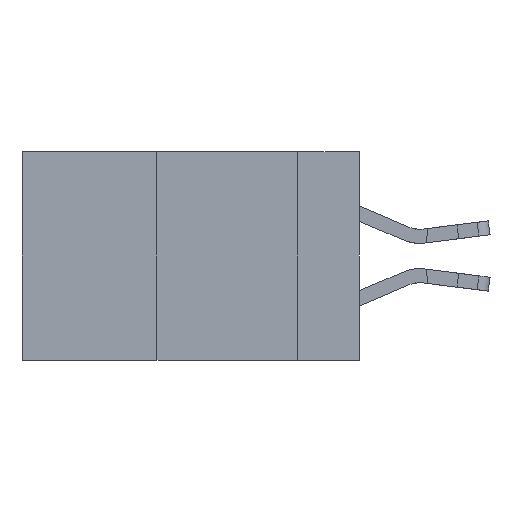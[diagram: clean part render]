
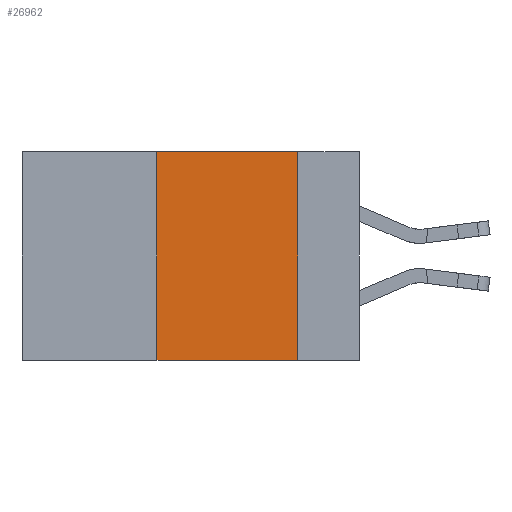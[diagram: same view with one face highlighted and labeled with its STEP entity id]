
A CAD part, left-side view. The second image highlights one B-rep face of the part: STEP entity #26962.
In plain terms, the highlighted planar face has unit normal (-1, 0, 0).
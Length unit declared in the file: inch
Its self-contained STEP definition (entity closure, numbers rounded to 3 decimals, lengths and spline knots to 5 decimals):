
#1200 = AXIS2_PLACEMENT_3D ( 'NONE', #20903, #7798, #16596 ) ;
#1503 = EDGE_CURVE ( 'NONE', #26457, #20012, #9806, .T. ) ;
#1635 = ORIENTED_EDGE ( 'NONE', *, *, #24283, .F. ) ;
#1770 = VERTEX_POINT ( 'NONE', #17729 ) ;
#2161 = VECTOR ( 'NONE', #19448, 39.37008 ) ;
#4522 = CARTESIAN_POINT ( 'NONE',  ( 0., 0.11, 0. ) ) ;
#4540 = LINE ( 'NONE', #4522, #2161 ) ;
#4823 = ORIENTED_EDGE ( 'NONE', *, *, #1503, .F. ) ;
#4982 = DIRECTION ( 'NONE',  ( 0., -1., 0. ) ) ;
#6367 = CARTESIAN_POINT ( 'NONE',  ( 0., 0.36, 0. ) ) ;
#6585 = FACE_OUTER_BOUND ( 'NONE', #18475, .T. ) ;
#7026 = DIRECTION ( 'NONE',  ( 0., -1., 0. ) ) ;
#7184 = LINE ( 'NONE', #13814, #11283 ) ;
#7602 = CARTESIAN_POINT ( 'NONE',  ( 0., 0.11, -0.37 ) ) ;
#7798 = DIRECTION ( 'NONE',  ( 1., 0., 0. ) ) ;
#7933 = ORIENTED_EDGE ( 'NONE', *, *, #28027, .T. ) ;
#9806 = LINE ( 'NONE', #12506, #13583 ) ;
#11283 = VECTOR ( 'NONE', #7026, 39.37008 ) ;
#12506 = CARTESIAN_POINT ( 'NONE',  ( 0., 0.36, 0. ) ) ;
#12717 = VECTOR ( 'NONE', #4982, 39.37008 ) ;
#13583 = VECTOR ( 'NONE', #21017, 39.37008 ) ;
#13814 = CARTESIAN_POINT ( 'NONE',  ( 0., 0.6, 0. ) ) ;
#15547 = VERTEX_POINT ( 'NONE', #7602 ) ;
#16596 = DIRECTION ( 'NONE',  ( 0., 0., -1. ) ) ;
#16908 = CARTESIAN_POINT ( 'NONE',  ( 0., 0.36, -0.37 ) ) ;
#17729 = CARTESIAN_POINT ( 'NONE',  ( 0., 0.11, 0. ) ) ;
#18475 = EDGE_LOOP ( 'NONE', ( #20619, #1635, #4823, #7933 ) ) ;
#19448 = DIRECTION ( 'NONE',  ( 0., 0., -1. ) ) ;
#20012 = VERTEX_POINT ( 'NONE', #6367 ) ;
#20568 = LINE ( 'NONE', #27107, #12717 ) ;
#20619 = ORIENTED_EDGE ( 'NONE', *, *, #22199, .F. ) ;
#20903 = CARTESIAN_POINT ( 'NONE',  ( 0., 0.6, 0. ) ) ;
#21017 = DIRECTION ( 'NONE',  ( 0., 0., 1. ) ) ;
#22199 = EDGE_CURVE ( 'NONE', #1770, #15547, #4540, .T. ) ;
#24283 = EDGE_CURVE ( 'NONE', #20012, #1770, #7184, .T. ) ;
#25332 = PLANE ( 'NONE',  #1200 ) ;
#26457 = VERTEX_POINT ( 'NONE', #16908 ) ;
#26962 = ADVANCED_FACE ( 'NONE', ( #6585 ), #25332, .F. ) ;
#27107 = CARTESIAN_POINT ( 'NONE',  ( 0., 0.6, -0.37 ) ) ;
#28027 = EDGE_CURVE ( 'NONE', #26457, #15547, #20568, .T. ) ;
